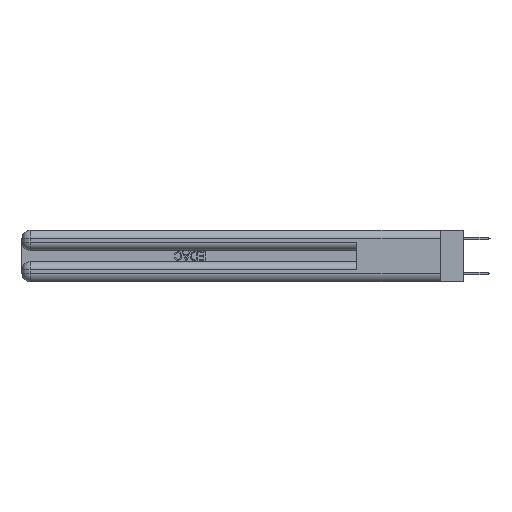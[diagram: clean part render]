
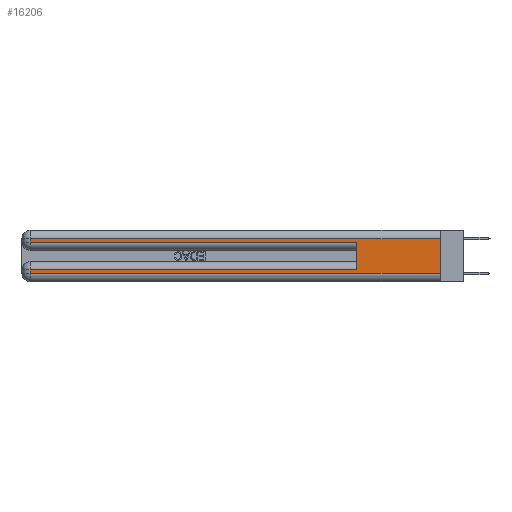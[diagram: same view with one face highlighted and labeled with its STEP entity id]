
A CAD part, left-side view. The second image highlights one B-rep face of the part: STEP entity #16206.
In plain terms, the highlighted planar face has unit normal (-1, 0, 0).
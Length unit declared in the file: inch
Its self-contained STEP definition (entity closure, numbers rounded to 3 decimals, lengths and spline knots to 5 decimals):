
#192 = LINE ( 'NONE', #32413, #6066 ) ;
#417 = ORIENTED_EDGE ( 'NONE', *, *, #6312, .T. ) ;
#787 = CARTESIAN_POINT ( 'NONE',  ( 0., 0.6, 0.145 ) ) ;
#1863 = DIRECTION ( 'NONE',  ( 0., 0., -1. ) ) ;
#2201 = VERTEX_POINT ( 'NONE', #22122 ) ;
#2240 = DIRECTION ( 'NONE',  ( 0., 0., -1. ) ) ;
#3135 = ORIENTED_EDGE ( 'NONE', *, *, #16514, .T. ) ;
#3152 = EDGE_CURVE ( 'NONE', #25087, #36213, #35248, .T. ) ;
#3489 = CARTESIAN_POINT ( 'NONE',  ( 0., 0., 0.285 ) ) ;
#3874 = LINE ( 'NONE', #29383, #10611 ) ;
#4074 = ORIENTED_EDGE ( 'NONE', *, *, #11578, .T. ) ;
#6066 = VECTOR ( 'NONE', #15606, 39.37008 ) ;
#6312 = EDGE_CURVE ( 'NONE', #35021, #2201, #7885, .T. ) ;
#7129 = ORIENTED_EDGE ( 'NONE', *, *, #16293, .F. ) ;
#7436 = LINE ( 'NONE', #19262, #24227 ) ;
#7539 = CARTESIAN_POINT ( 'NONE',  ( 0., 0., 0.37 ) ) ;
#7870 = VECTOR ( 'NONE', #20469, 39.37008 ) ;
#7885 = LINE ( 'NONE', #13269, #14522 ) ;
#8274 = VERTEX_POINT ( 'NONE', #23253 ) ;
#9675 = DIRECTION ( 'NONE',  ( 0., -1., 0. ) ) ;
#10611 = VECTOR ( 'NONE', #9675, 39.37008 ) ;
#10925 = CARTESIAN_POINT ( 'NONE',  ( 0., 0., 0.06 ) ) ;
#11578 = EDGE_CURVE ( 'NONE', #34059, #29606, #3874, .T. ) ;
#11911 = FACE_OUTER_BOUND ( 'NONE', #27993, .T. ) ;
#12554 = CARTESIAN_POINT ( 'NONE',  ( 0., 0., 0.31 ) ) ;
#13261 = PLANE ( 'NONE',  #26657 ) ;
#13269 = CARTESIAN_POINT ( 'NONE',  ( 0., 2.94, 0.37 ) ) ;
#13395 = VECTOR ( 'NONE', #34273, 39.37008 ) ;
#13446 = EDGE_CURVE ( 'NONE', #32113, #34059, #192, .T. ) ;
#13940 = EDGE_CURVE ( 'NONE', #8274, #35021, #26801, .T. ) ;
#14045 = CARTESIAN_POINT ( 'NONE',  ( 0., 2.94, 0.31 ) ) ;
#14522 = VECTOR ( 'NONE', #1863, 39.37008 ) ;
#14561 = CARTESIAN_POINT ( 'NONE',  ( 0., 2.94, 0.06 ) ) ;
#15606 = DIRECTION ( 'NONE',  ( 0., 0., -1. ) ) ;
#16076 = DIRECTION ( 'NONE',  ( 0., 0., -1. ) ) ;
#16206 = ADVANCED_FACE ( 'NONE', ( #11911 ), #13261, .F. ) ;
#16293 = EDGE_CURVE ( 'NONE', #8274, #29606, #7436, .T. ) ;
#16514 = EDGE_CURVE ( 'NONE', #2201, #36213, #22879, .T. ) ;
#17548 = ORIENTED_EDGE ( 'NONE', *, *, #34103, .T. ) ;
#18434 = ORIENTED_EDGE ( 'NONE', *, *, #3152, .F. ) ;
#18538 = CARTESIAN_POINT ( 'NONE',  ( 0., 0.6, 0.085 ) ) ;
#19262 = CARTESIAN_POINT ( 'NONE',  ( 0., 0., 0.37 ) ) ;
#20469 = DIRECTION ( 'NONE',  ( 0., -1., 0. ) ) ;
#21757 = LINE ( 'NONE', #28722, #13395 ) ;
#22088 = CARTESIAN_POINT ( 'NONE',  ( 0., 0.6, 0.285 ) ) ;
#22122 = CARTESIAN_POINT ( 'NONE',  ( 0., 2.94, 0.285 ) ) ;
#22378 = ORIENTED_EDGE ( 'NONE', *, *, #13940, .T. ) ;
#22879 = LINE ( 'NONE', #3489, #7870 ) ;
#23253 = CARTESIAN_POINT ( 'NONE',  ( 0., 0., 0.31 ) ) ;
#24227 = VECTOR ( 'NONE', #2240, 39.37008 ) ;
#25087 = VERTEX_POINT ( 'NONE', #18538 ) ;
#25921 = VECTOR ( 'NONE', #29393, 39.37008 ) ;
#26657 = AXIS2_PLACEMENT_3D ( 'NONE', #7539, #32867, #16076 ) ;
#26801 = LINE ( 'NONE', #12554, #25921 ) ;
#27891 = VECTOR ( 'NONE', #29185, 39.37008 ) ;
#27993 = EDGE_LOOP ( 'NONE', ( #7129, #22378, #417, #3135, #18434, #17548, #30657, #4074 ) ) ;
#28722 = CARTESIAN_POINT ( 'NONE',  ( 0., 0., 0.085 ) ) ;
#29185 = DIRECTION ( 'NONE',  ( 0., 0., 1. ) ) ;
#29383 = CARTESIAN_POINT ( 'NONE',  ( 0., 0., 0.06 ) ) ;
#29393 = DIRECTION ( 'NONE',  ( 0., 1., 0. ) ) ;
#29606 = VERTEX_POINT ( 'NONE', #10925 ) ;
#30657 = ORIENTED_EDGE ( 'NONE', *, *, #13446, .T. ) ;
#31159 = CARTESIAN_POINT ( 'NONE',  ( 0., 2.94, 0.085 ) ) ;
#32113 = VERTEX_POINT ( 'NONE', #31159 ) ;
#32413 = CARTESIAN_POINT ( 'NONE',  ( 0., 2.94, 0.37 ) ) ;
#32867 = DIRECTION ( 'NONE',  ( 1., 0., 0. ) ) ;
#34059 = VERTEX_POINT ( 'NONE', #14561 ) ;
#34103 = EDGE_CURVE ( 'NONE', #25087, #32113, #21757, .T. ) ;
#34273 = DIRECTION ( 'NONE',  ( 0., 1., 0. ) ) ;
#35021 = VERTEX_POINT ( 'NONE', #14045 ) ;
#35248 = LINE ( 'NONE', #787, #27891 ) ;
#36213 = VERTEX_POINT ( 'NONE', #22088 ) ;
